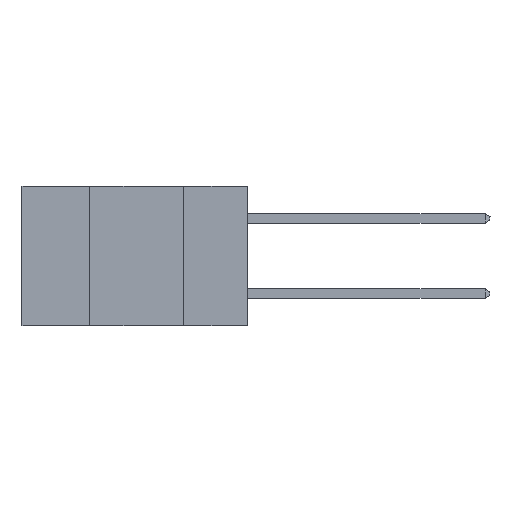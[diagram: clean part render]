
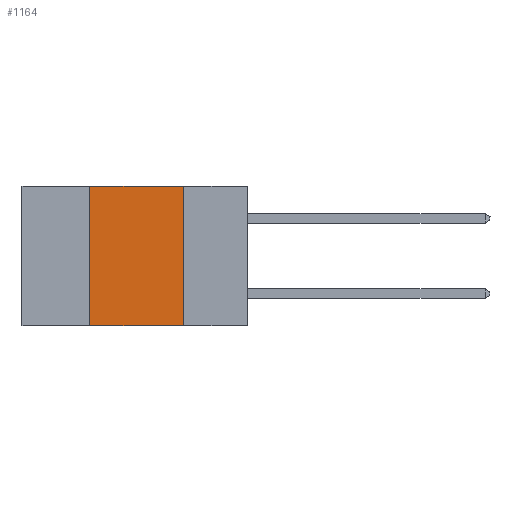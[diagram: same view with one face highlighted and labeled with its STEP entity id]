
A CAD part, left-side view. The second image highlights one B-rep face of the part: STEP entity #1164.
In plain terms, the highlighted planar face has unit normal (-1, 0, 0).
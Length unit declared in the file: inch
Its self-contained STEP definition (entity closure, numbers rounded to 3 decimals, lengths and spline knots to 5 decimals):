
#606 = LINE ( 'NONE', #8216, #8860 ) ;
#694 = EDGE_CURVE ( 'NONE', #7494, #1172, #3443, .T. ) ;
#1164 = ADVANCED_FACE ( 'NONE', ( #7138 ), #13685, .F. ) ;
#1172 = VERTEX_POINT ( 'NONE', #2866 ) ;
#1572 = LINE ( 'NONE', #2771, #11499 ) ;
#2760 = VERTEX_POINT ( 'NONE', #12214 ) ;
#2771 = CARTESIAN_POINT ( 'NONE',  ( 0., 0.17, -0.37 ) ) ;
#2866 = CARTESIAN_POINT ( 'NONE',  ( 0., 0.42, 0. ) ) ;
#2916 = LINE ( 'NONE', #11646, #6014 ) ;
#3443 = LINE ( 'NONE', #6929, #9576 ) ;
#4882 = ORIENTED_EDGE ( 'NONE', *, *, #694, .F. ) ;
#5267 = ORIENTED_EDGE ( 'NONE', *, *, #8621, .F. ) ;
#5898 = DIRECTION ( 'NONE',  ( 0., 0., -1. ) ) ;
#5981 = ORIENTED_EDGE ( 'NONE', *, *, #9385, .F. ) ;
#6014 = VECTOR ( 'NONE', #10424, 39.37008 ) ;
#6206 = ORIENTED_EDGE ( 'NONE', *, *, #11587, .T. ) ;
#6625 = AXIS2_PLACEMENT_3D ( 'NONE', #13482, #6989, #7280 ) ;
#6929 = CARTESIAN_POINT ( 'NONE',  ( 0., 0.42, -0.37 ) ) ;
#6989 = DIRECTION ( 'NONE',  ( 1., 0., 0. ) ) ;
#7138 = FACE_OUTER_BOUND ( 'NONE', #9420, .T. ) ;
#7266 = VERTEX_POINT ( 'NONE', #7709 ) ;
#7280 = DIRECTION ( 'NONE',  ( 0., 0., -1. ) ) ;
#7494 = VERTEX_POINT ( 'NONE', #10929 ) ;
#7709 = CARTESIAN_POINT ( 'NONE',  ( 0., 0.17, 0. ) ) ;
#8216 = CARTESIAN_POINT ( 'NONE',  ( 0., 0.6, -0.37 ) ) ;
#8621 = EDGE_CURVE ( 'NONE', #7266, #2760, #1572, .T. ) ;
#8860 = VECTOR ( 'NONE', #12532, 39.37008 ) ;
#9385 = EDGE_CURVE ( 'NONE', #1172, #7266, #2916, .T. ) ;
#9420 = EDGE_LOOP ( 'NONE', ( #5267, #5981, #4882, #6206 ) ) ;
#9576 = VECTOR ( 'NONE', #12163, 39.37008 ) ;
#10424 = DIRECTION ( 'NONE',  ( 0., -1., 0. ) ) ;
#10929 = CARTESIAN_POINT ( 'NONE',  ( 0., 0.42, -0.37 ) ) ;
#11499 = VECTOR ( 'NONE', #5898, 39.37008 ) ;
#11587 = EDGE_CURVE ( 'NONE', #7494, #2760, #606, .T. ) ;
#11646 = CARTESIAN_POINT ( 'NONE',  ( 0., 0.6, 0. ) ) ;
#12163 = DIRECTION ( 'NONE',  ( 0., 0., 1. ) ) ;
#12214 = CARTESIAN_POINT ( 'NONE',  ( 0., 0.17, -0.37 ) ) ;
#12532 = DIRECTION ( 'NONE',  ( 0., -1., 0. ) ) ;
#13482 = CARTESIAN_POINT ( 'NONE',  ( 0., 0.6, 0. ) ) ;
#13685 = PLANE ( 'NONE',  #6625 ) ;
